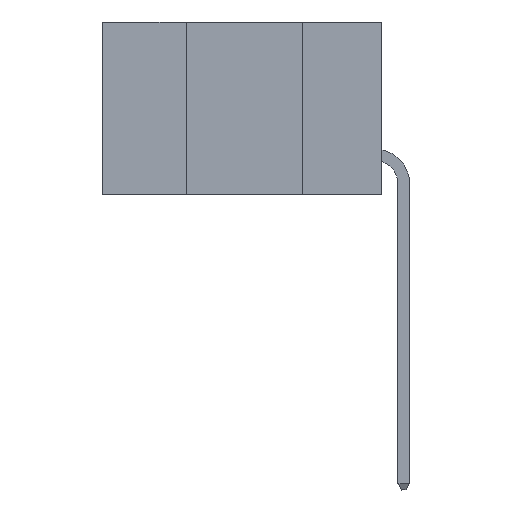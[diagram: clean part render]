
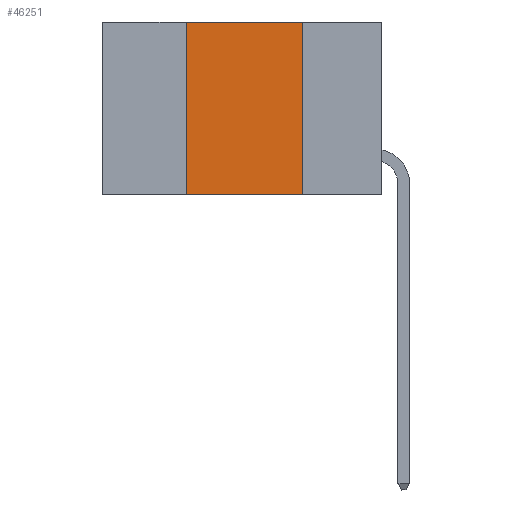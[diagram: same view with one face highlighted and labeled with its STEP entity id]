
A CAD part, left-side view. The second image highlights one B-rep face of the part: STEP entity #46251.
In plain terms, the highlighted planar face has unit normal (-1, 0, 0).
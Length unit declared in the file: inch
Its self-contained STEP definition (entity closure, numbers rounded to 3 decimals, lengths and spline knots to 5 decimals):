
#530 = LINE ( 'NONE', #2147, #29823 ) ;
#2147 = CARTESIAN_POINT ( 'NONE',  ( 0., 0.6, -0.37 ) ) ;
#4882 = CARTESIAN_POINT ( 'NONE',  ( 0., 0.6, 0. ) ) ;
#8334 = ORIENTED_EDGE ( 'NONE', *, *, #15169, .F. ) ;
#9148 = FACE_OUTER_BOUND ( 'NONE', #30431, .T. ) ;
#11119 = EDGE_CURVE ( 'NONE', #40487, #34869, #28428, .T. ) ;
#12505 = VERTEX_POINT ( 'NONE', #18693 ) ;
#15169 = EDGE_CURVE ( 'NONE', #34869, #12505, #48901, .T. ) ;
#16067 = CARTESIAN_POINT ( 'NONE',  ( 0., 0.17, 0. ) ) ;
#18693 = CARTESIAN_POINT ( 'NONE',  ( 0., 0.17, 0. ) ) ;
#19263 = VECTOR ( 'NONE', #23389, 39.37008 ) ;
#21780 = CARTESIAN_POINT ( 'NONE',  ( 0., 0.6, 0. ) ) ;
#21949 = DIRECTION ( 'NONE',  ( 1., 0., 0. ) ) ;
#23389 = DIRECTION ( 'NONE',  ( 0., 0., -1. ) ) ;
#23819 = ORIENTED_EDGE ( 'NONE', *, *, #11119, .F. ) ;
#25576 = CARTESIAN_POINT ( 'NONE',  ( 0., 0.17, -0.37 ) ) ;
#25818 = PLANE ( 'NONE',  #29110 ) ;
#28428 = LINE ( 'NONE', #32925, #38987 ) ;
#29110 = AXIS2_PLACEMENT_3D ( 'NONE', #21780, #21949, #37634 ) ;
#29454 = DIRECTION ( 'NONE',  ( 0., 0., 1. ) ) ;
#29501 = ORIENTED_EDGE ( 'NONE', *, *, #41708, .F. ) ;
#29823 = VECTOR ( 'NONE', #42153, 39.37008 ) ;
#30431 = EDGE_LOOP ( 'NONE', ( #29501, #8334, #23819, #40974 ) ) ;
#32925 = CARTESIAN_POINT ( 'NONE',  ( 0., 0.42, 0. ) ) ;
#34869 = VERTEX_POINT ( 'NONE', #38976 ) ;
#37634 = DIRECTION ( 'NONE',  ( 0., 0., -1. ) ) ;
#38976 = CARTESIAN_POINT ( 'NONE',  ( 0., 0.42, 0. ) ) ;
#38987 = VECTOR ( 'NONE', #29454, 39.37008 ) ;
#40408 = LINE ( 'NONE', #16067, #19263 ) ;
#40487 = VERTEX_POINT ( 'NONE', #44276 ) ;
#40974 = ORIENTED_EDGE ( 'NONE', *, *, #42168, .T. ) ;
#41708 = EDGE_CURVE ( 'NONE', #12505, #49616, #40408, .T. ) ;
#42153 = DIRECTION ( 'NONE',  ( 0., -1., 0. ) ) ;
#42168 = EDGE_CURVE ( 'NONE', #40487, #49616, #530, .T. ) ;
#44276 = CARTESIAN_POINT ( 'NONE',  ( 0., 0.42, -0.37 ) ) ;
#44537 = DIRECTION ( 'NONE',  ( 0., -1., 0. ) ) ;
#46251 = ADVANCED_FACE ( 'NONE', ( #9148 ), #25818, .F. ) ;
#48901 = LINE ( 'NONE', #4882, #51396 ) ;
#49616 = VERTEX_POINT ( 'NONE', #25576 ) ;
#51396 = VECTOR ( 'NONE', #44537, 39.37008 ) ;
